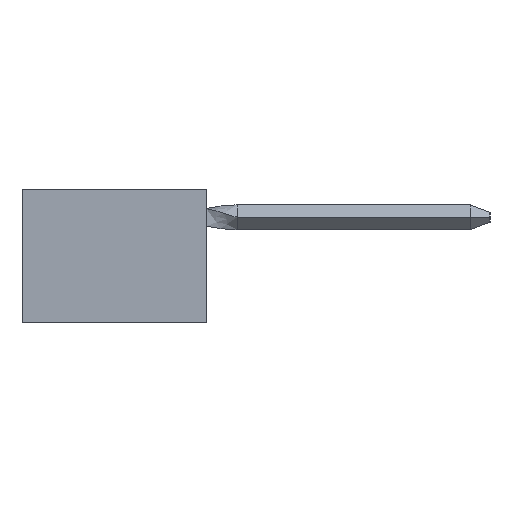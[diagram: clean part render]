
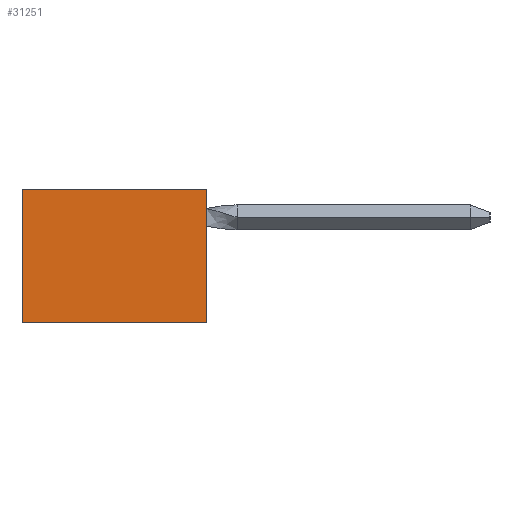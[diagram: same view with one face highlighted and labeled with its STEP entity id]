
A CAD part, left-side view. The second image highlights one B-rep face of the part: STEP entity #31251.
In plain terms, the highlighted planar face has unit normal (-1, 0, 0).
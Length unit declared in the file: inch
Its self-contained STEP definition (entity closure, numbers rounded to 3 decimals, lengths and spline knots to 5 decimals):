
#1219 = EDGE_CURVE ( 'NONE', #21310, #35041, #48083, .T. ) ;
#2247 = PLANE ( 'NONE',  #3036 ) ;
#2435 = CARTESIAN_POINT ( 'NONE',  ( 0.298, -0.027, 0. ) ) ;
#2549 = VECTOR ( 'NONE', #16251, 39.37008 ) ;
#3036 = AXIS2_PLACEMENT_3D ( 'NONE', #2435, #40029, #31538 ) ;
#4261 = VERTEX_POINT ( 'NONE', #43089 ) ;
#4746 = VERTEX_POINT ( 'NONE', #27201 ) ;
#13449 = CARTESIAN_POINT ( 'NONE',  ( 0.298, 0.473, -0.343 ) ) ;
#16251 = DIRECTION ( 'NONE',  ( 0., 0., 1. ) ) ;
#20215 = ORIENTED_EDGE ( 'NONE', *, *, #1219, .T. ) ;
#20360 = VECTOR ( 'NONE', #40626, 39.37008 ) ;
#21310 = VERTEX_POINT ( 'NONE', #29886 ) ;
#24900 = ORIENTED_EDGE ( 'NONE', *, *, #27808, .T. ) ;
#26666 = CARTESIAN_POINT ( 'NONE',  ( 0.298, 0., 0. ) ) ;
#27201 = CARTESIAN_POINT ( 'NONE',  ( 0.298, 0.473, -0.343 ) ) ;
#27808 = EDGE_CURVE ( 'NONE', #35041, #4261, #31641, .T. ) ;
#29886 = CARTESIAN_POINT ( 'NONE',  ( 0.298, 0., -0.343 ) ) ;
#30393 = EDGE_CURVE ( 'NONE', #21310, #4746, #31674, .T. ) ;
#31251 = ADVANCED_FACE ( 'NONE', ( #38202 ), #2247, .F. ) ;
#31538 = DIRECTION ( 'NONE',  ( 0., 0., -1. ) ) ;
#31641 = LINE ( 'NONE', #53450, #20360 ) ;
#31674 = LINE ( 'NONE', #13449, #52892 ) ;
#35041 = VERTEX_POINT ( 'NONE', #26666 ) ;
#35479 = CARTESIAN_POINT ( 'NONE',  ( 0.298, 0.473, 0. ) ) ;
#35781 = EDGE_CURVE ( 'NONE', #4261, #4746, #51022, .T. ) ;
#38202 = FACE_OUTER_BOUND ( 'NONE', #41252, .T. ) ;
#40029 = DIRECTION ( 'NONE',  ( 1., 0., 0. ) ) ;
#40626 = DIRECTION ( 'NONE',  ( 0., 1., 0. ) ) ;
#40734 = ORIENTED_EDGE ( 'NONE', *, *, #30393, .F. ) ;
#41090 = VECTOR ( 'NONE', #49762, 39.37008 ) ;
#41252 = EDGE_LOOP ( 'NONE', ( #20215, #24900, #53839, #40734 ) ) ;
#43080 = DIRECTION ( 'NONE',  ( 0., 1., 0. ) ) ;
#43089 = CARTESIAN_POINT ( 'NONE',  ( 0.298, 0.473, 0. ) ) ;
#46434 = CARTESIAN_POINT ( 'NONE',  ( 0.298, 0., -0.343 ) ) ;
#48083 = LINE ( 'NONE', #46434, #2549 ) ;
#49762 = DIRECTION ( 'NONE',  ( 0., 0., -1. ) ) ;
#51022 = LINE ( 'NONE', #35479, #41090 ) ;
#52892 = VECTOR ( 'NONE', #43080, 39.37008 ) ;
#53450 = CARTESIAN_POINT ( 'NONE',  ( 0.298, -0.027, 0. ) ) ;
#53839 = ORIENTED_EDGE ( 'NONE', *, *, #35781, .T. ) ;
